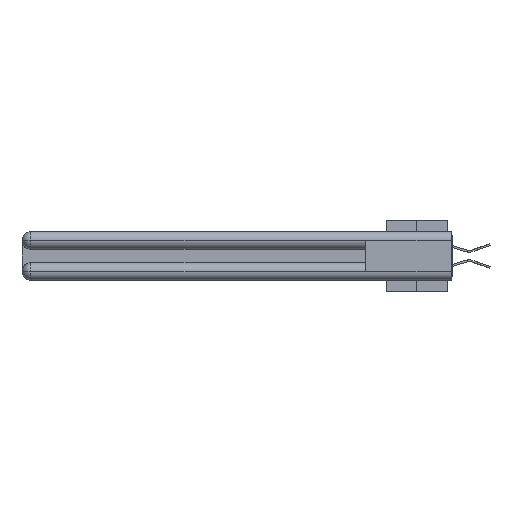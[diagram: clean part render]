
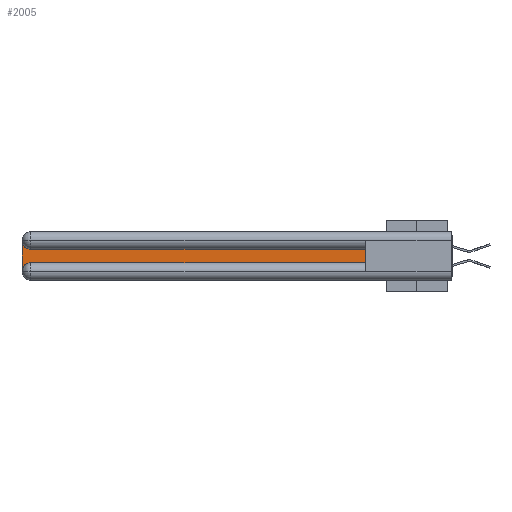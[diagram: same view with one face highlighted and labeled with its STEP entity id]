
A CAD part, left-side view. The second image highlights one B-rep face of the part: STEP entity #2005.
In plain terms, the highlighted planar face has unit normal (-1, 0, 0).
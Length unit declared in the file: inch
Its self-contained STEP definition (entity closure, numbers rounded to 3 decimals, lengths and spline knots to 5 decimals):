
#342 = FACE_OUTER_BOUND ( 'NONE', #17981, .T. ) ;
#359 = EDGE_CURVE ( 'NONE', #7051, #2615, #38246, .T. ) ;
#587 = ORIENTED_EDGE ( 'NONE', *, *, #32064, .T. ) ;
#845 = CARTESIAN_POINT ( 'NONE',  ( 0.075, 0.6, -0.2175 ) ) ;
#902 = PLANE ( 'NONE',  #19783 ) ;
#2005 = ADVANCED_FACE ( 'NONE', ( #342 ), #902, .F. ) ;
#2615 = VERTEX_POINT ( 'NONE', #42103 ) ;
#5666 = CIRCLE ( 'NONE', #17429, 0.06 ) ;
#6105 = CIRCLE ( 'NONE', #25180, 0.06 ) ;
#6958 = EDGE_CURVE ( 'NONE', #2615, #19900, #6105, .T. ) ;
#7051 = VERTEX_POINT ( 'NONE', #18344 ) ;
#7164 = VECTOR ( 'NONE', #24038, 39.37008 ) ;
#7838 = CARTESIAN_POINT ( 'NONE',  ( 0.075, 3., -0.2175 ) ) ;
#8238 = ORIENTED_EDGE ( 'NONE', *, *, #6958, .T. ) ;
#9349 = VERTEX_POINT ( 'NONE', #28760 ) ;
#10588 = CARTESIAN_POINT ( 'NONE',  ( 0.075, 0.6, -0.2175 ) ) ;
#10854 = CARTESIAN_POINT ( 'NONE',  ( 0.075, 3., -0.1225 ) ) ;
#11124 = VECTOR ( 'NONE', #17063, 39.37008 ) ;
#11274 = DIRECTION ( 'NONE',  ( 1., 0., 0. ) ) ;
#11934 = VERTEX_POINT ( 'NONE', #24058 ) ;
#12615 = DIRECTION ( 'NONE',  ( 0., 0., -1. ) ) ;
#14640 = DIRECTION ( 'NONE',  ( 0., 0., -1. ) ) ;
#15810 = ORIENTED_EDGE ( 'NONE', *, *, #359, .T. ) ;
#16641 = LINE ( 'NONE', #845, #32436 ) ;
#16810 = ORIENTED_EDGE ( 'NONE', *, *, #22622, .T. ) ;
#17063 = DIRECTION ( 'NONE',  ( 0., 1., 0. ) ) ;
#17429 = AXIS2_PLACEMENT_3D ( 'NONE', #22863, #33389, #12615 ) ;
#17981 = EDGE_LOOP ( 'NONE', ( #15810, #8238, #16810, #38919, #587, #20941 ) ) ;
#18080 = DIRECTION ( 'NONE',  ( 1., 0., 0. ) ) ;
#18344 = CARTESIAN_POINT ( 'NONE',  ( 0.075, 0.6, -0.1225 ) ) ;
#18661 = DIRECTION ( 'NONE',  ( 0., 0., -1. ) ) ;
#19783 = AXIS2_PLACEMENT_3D ( 'NONE', #10854, #18080, #14640 ) ;
#19900 = VERTEX_POINT ( 'NONE', #42016 ) ;
#20941 = ORIENTED_EDGE ( 'NONE', *, *, #28409, .T. ) ;
#21407 = DIRECTION ( 'NONE',  ( 0., 0., -1. ) ) ;
#22622 = EDGE_CURVE ( 'NONE', #19900, #11934, #35768, .T. ) ;
#22863 = CARTESIAN_POINT ( 'NONE',  ( 0.075, 2.94, -0.2775 ) ) ;
#24038 = DIRECTION ( 'NONE',  ( 0., -1., 0. ) ) ;
#24058 = CARTESIAN_POINT ( 'NONE',  ( 0.075, 3., -0.2775 ) ) ;
#24636 = EDGE_CURVE ( 'NONE', #11934, #9349, #5666, .T. ) ;
#24690 = DIRECTION ( 'NONE',  ( 0., 0., 1. ) ) ;
#25180 = AXIS2_PLACEMENT_3D ( 'NONE', #31117, #11274, #21407 ) ;
#25361 = VECTOR ( 'NONE', #18661, 39.37008 ) ;
#28409 = EDGE_CURVE ( 'NONE', #29761, #7051, #16641, .T. ) ;
#28760 = CARTESIAN_POINT ( 'NONE',  ( 0.075, 2.94, -0.2175 ) ) ;
#29761 = VERTEX_POINT ( 'NONE', #44644 ) ;
#31117 = CARTESIAN_POINT ( 'NONE',  ( 0.075, 2.94, -0.0625 ) ) ;
#32064 = EDGE_CURVE ( 'NONE', #9349, #29761, #40256, .T. ) ;
#32436 = VECTOR ( 'NONE', #24690, 39.37008 ) ;
#33389 = DIRECTION ( 'NONE',  ( 1., 0., 0. ) ) ;
#35768 = LINE ( 'NONE', #7838, #25361 ) ;
#38246 = LINE ( 'NONE', #41376, #11124 ) ;
#38919 = ORIENTED_EDGE ( 'NONE', *, *, #24636, .T. ) ;
#40256 = LINE ( 'NONE', #10588, #7164 ) ;
#41376 = CARTESIAN_POINT ( 'NONE',  ( 0.075, 0.6, -0.1225 ) ) ;
#42016 = CARTESIAN_POINT ( 'NONE',  ( 0.075, 3., -0.0625 ) ) ;
#42103 = CARTESIAN_POINT ( 'NONE',  ( 0.075, 2.94, -0.1225 ) ) ;
#44644 = CARTESIAN_POINT ( 'NONE',  ( 0.075, 0.6, -0.2175 ) ) ;
